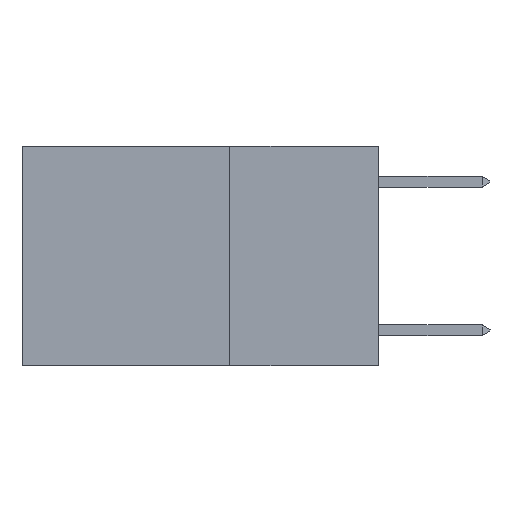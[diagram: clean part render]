
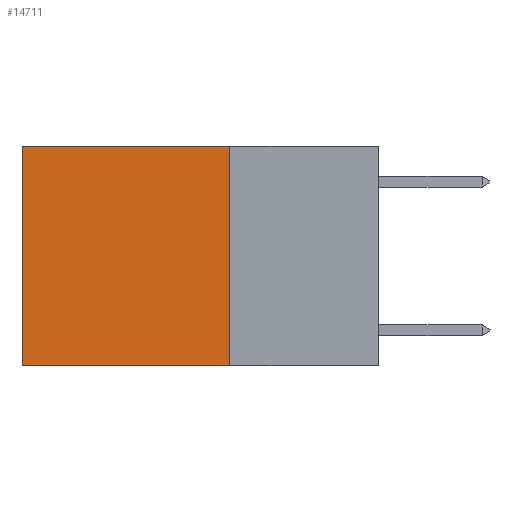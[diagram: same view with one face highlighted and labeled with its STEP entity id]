
A CAD part, left-side view. The second image highlights one B-rep face of the part: STEP entity #14711.
In plain terms, the highlighted planar face has unit normal (-1, 0, 0).
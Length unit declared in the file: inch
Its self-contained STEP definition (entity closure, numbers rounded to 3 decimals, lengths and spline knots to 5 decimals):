
#2024 = EDGE_CURVE ( 'NONE', #12361, #28151, #13405, .T. ) ;
#3237 = DIRECTION ( 'NONE',  ( 0., 0., -1. ) ) ;
#3442 = CARTESIAN_POINT ( 'NONE',  ( 0.2625, 0.25, -0.37 ) ) ;
#3779 = FACE_OUTER_BOUND ( 'NONE', #17247, .T. ) ;
#3952 = ORIENTED_EDGE ( 'NONE', *, *, #6464, .T. ) ;
#4055 = DIRECTION ( 'NONE',  ( 1., 0., 0. ) ) ;
#5231 = ORIENTED_EDGE ( 'NONE', *, *, #2024, .F. ) ;
#5806 = DIRECTION ( 'NONE',  ( 0., 1., 0. ) ) ;
#5984 = VECTOR ( 'NONE', #24904, 39.37008 ) ;
#6066 = CARTESIAN_POINT ( 'NONE',  ( 0.2625, 0.25, 0. ) ) ;
#6397 = CARTESIAN_POINT ( 'NONE',  ( 0.2625, 0.6, 0. ) ) ;
#6464 = EDGE_CURVE ( 'NONE', #12361, #18846, #7514, .T. ) ;
#7514 = LINE ( 'NONE', #6066, #5984 ) ;
#8928 = LINE ( 'NONE', #26779, #20847 ) ;
#10280 = VECTOR ( 'NONE', #5806, 39.37008 ) ;
#12361 = VERTEX_POINT ( 'NONE', #21319 ) ;
#13353 = VECTOR ( 'NONE', #3237, 39.37008 ) ;
#13405 = LINE ( 'NONE', #19852, #13353 ) ;
#14711 = ADVANCED_FACE ( 'NONE', ( #3779 ), #29747, .F. ) ;
#15786 = ORIENTED_EDGE ( 'NONE', *, *, #21070, .F. ) ;
#16585 = LINE ( 'NONE', #3442, #10280 ) ;
#17247 = EDGE_LOOP ( 'NONE', ( #26889, #15786, #5231, #3952 ) ) ;
#18306 = CARTESIAN_POINT ( 'NONE',  ( 0.2625, 0.25, 0. ) ) ;
#18846 = VERTEX_POINT ( 'NONE', #6397 ) ;
#19740 = CARTESIAN_POINT ( 'NONE',  ( 0.2625, 0.6, -0.37 ) ) ;
#19852 = CARTESIAN_POINT ( 'NONE',  ( 0.2625, 0.25, 0. ) ) ;
#20666 = DIRECTION ( 'NONE',  ( 0., 0., -1. ) ) ;
#20847 = VECTOR ( 'NONE', #29049, 39.37008 ) ;
#20996 = VERTEX_POINT ( 'NONE', #19740 ) ;
#21070 = EDGE_CURVE ( 'NONE', #28151, #20996, #16585, .T. ) ;
#21319 = CARTESIAN_POINT ( 'NONE',  ( 0.2625, 0.25, 0. ) ) ;
#21464 = AXIS2_PLACEMENT_3D ( 'NONE', #18306, #4055, #20666 ) ;
#24700 = EDGE_CURVE ( 'NONE', #18846, #20996, #8928, .T. ) ;
#24904 = DIRECTION ( 'NONE',  ( 0., 1., 0. ) ) ;
#26779 = CARTESIAN_POINT ( 'NONE',  ( 0.2625, 0.6, 0. ) ) ;
#26889 = ORIENTED_EDGE ( 'NONE', *, *, #24700, .T. ) ;
#28151 = VERTEX_POINT ( 'NONE', #29476 ) ;
#29049 = DIRECTION ( 'NONE',  ( 0., 0., -1. ) ) ;
#29476 = CARTESIAN_POINT ( 'NONE',  ( 0.2625, 0.25, -0.37 ) ) ;
#29747 = PLANE ( 'NONE',  #21464 ) ;
